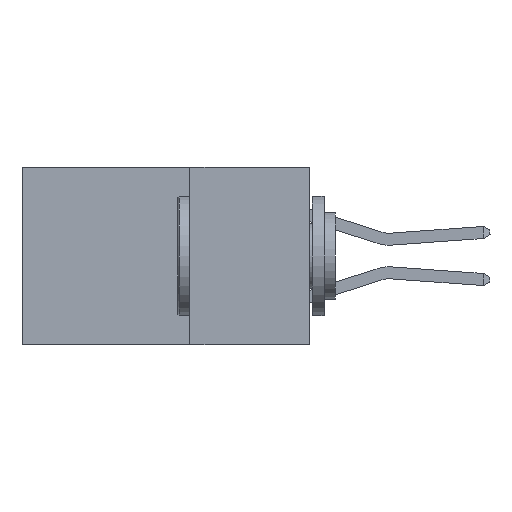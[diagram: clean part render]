
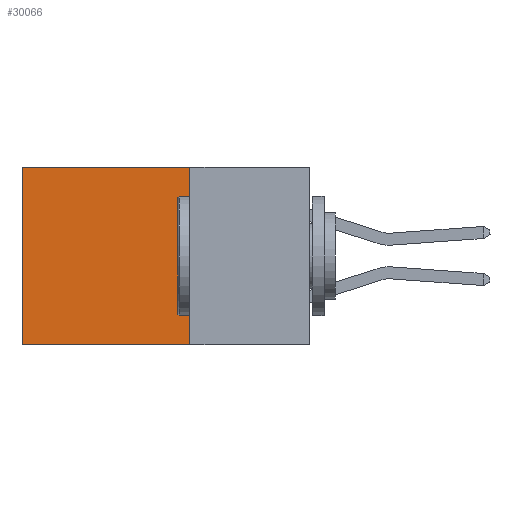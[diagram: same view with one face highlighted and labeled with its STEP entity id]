
A CAD part, left-side view. The second image highlights one B-rep face of the part: STEP entity #30066.
In plain terms, the highlighted planar face has unit normal (-1, 0, 0).
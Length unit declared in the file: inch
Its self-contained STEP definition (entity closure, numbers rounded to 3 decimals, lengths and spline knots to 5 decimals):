
#1632 = ORIENTED_EDGE ( 'NONE', *, *, #28387, .F. ) ;
#2041 = PLANE ( 'NONE',  #30103 ) ;
#3045 = FACE_OUTER_BOUND ( 'NONE', #29182, .T. ) ;
#3125 = EDGE_CURVE ( 'NONE', #18497, #20660, #13810, .T. ) ;
#3445 = DIRECTION ( 'NONE',  ( 0., 1., 0. ) ) ;
#5842 = CARTESIAN_POINT ( 'NONE',  ( 0.298, 0.6, 0. ) ) ;
#6647 = VECTOR ( 'NONE', #28535, 39.37008 ) ;
#7041 = DIRECTION ( 'NONE',  ( 1., 0., 0. ) ) ;
#7479 = LINE ( 'NONE', #13096, #18742 ) ;
#9216 = DIRECTION ( 'NONE',  ( 0., 1., 0. ) ) ;
#10033 = CARTESIAN_POINT ( 'NONE',  ( 0.298, 0.6, 0. ) ) ;
#13096 = CARTESIAN_POINT ( 'NONE',  ( 0.298, 0.25, -0.37 ) ) ;
#13810 = LINE ( 'NONE', #5842, #19451 ) ;
#14371 = EDGE_CURVE ( 'NONE', #25745, #18497, #24364, .T. ) ;
#17052 = ORIENTED_EDGE ( 'NONE', *, *, #14371, .T. ) ;
#18497 = VERTEX_POINT ( 'NONE', #10033 ) ;
#18742 = VECTOR ( 'NONE', #3445, 39.37008 ) ;
#19451 = VECTOR ( 'NONE', #19524, 39.37008 ) ;
#19455 = LINE ( 'NONE', #30916, #6647 ) ;
#19524 = DIRECTION ( 'NONE',  ( 0., 0., -1. ) ) ;
#20571 = CARTESIAN_POINT ( 'NONE',  ( 0.298, 0.6, -0.37 ) ) ;
#20660 = VERTEX_POINT ( 'NONE', #20571 ) ;
#20745 = EDGE_CURVE ( 'NONE', #24156, #20660, #7479, .T. ) ;
#21462 = CARTESIAN_POINT ( 'NONE',  ( 0.298, 0.25, 0. ) ) ;
#21598 = ORIENTED_EDGE ( 'NONE', *, *, #20745, .F. ) ;
#22098 = CARTESIAN_POINT ( 'NONE',  ( 0.298, 0.25, -0.37 ) ) ;
#22854 = VECTOR ( 'NONE', #9216, 39.37008 ) ;
#23878 = DIRECTION ( 'NONE',  ( 0., 0., -1. ) ) ;
#24023 = ORIENTED_EDGE ( 'NONE', *, *, #3125, .T. ) ;
#24156 = VERTEX_POINT ( 'NONE', #22098 ) ;
#24364 = LINE ( 'NONE', #28514, #22854 ) ;
#25745 = VERTEX_POINT ( 'NONE', #28275 ) ;
#28275 = CARTESIAN_POINT ( 'NONE',  ( 0.298, 0.25, 0. ) ) ;
#28387 = EDGE_CURVE ( 'NONE', #25745, #24156, #19455, .T. ) ;
#28514 = CARTESIAN_POINT ( 'NONE',  ( 0.298, 0.25, 0. ) ) ;
#28535 = DIRECTION ( 'NONE',  ( 0., 0., -1. ) ) ;
#29182 = EDGE_LOOP ( 'NONE', ( #24023, #21598, #1632, #17052 ) ) ;
#30066 = ADVANCED_FACE ( 'NONE', ( #3045 ), #2041, .F. ) ;
#30103 = AXIS2_PLACEMENT_3D ( 'NONE', #21462, #7041, #23878 ) ;
#30916 = CARTESIAN_POINT ( 'NONE',  ( 0.298, 0.25, 0. ) ) ;
